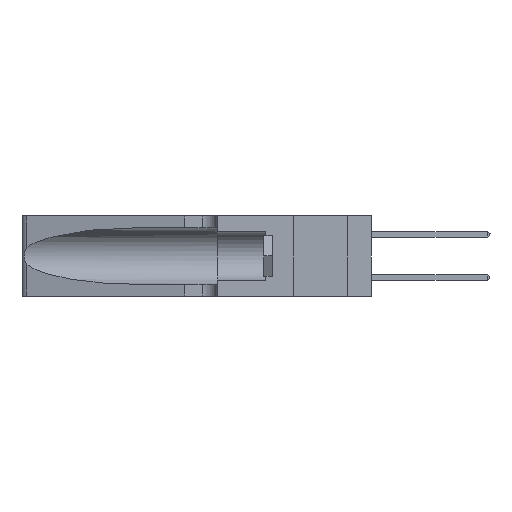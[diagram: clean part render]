
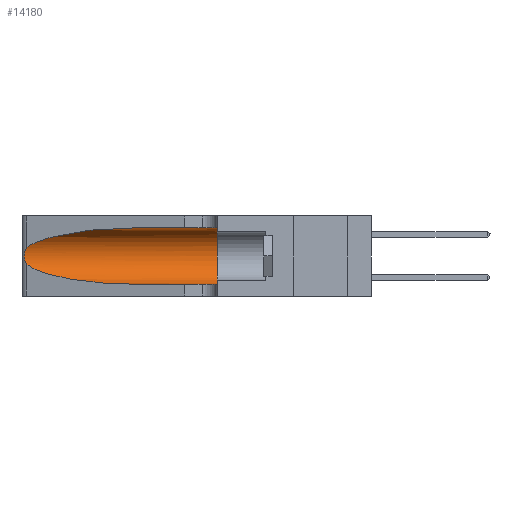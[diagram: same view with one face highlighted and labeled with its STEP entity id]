
A CAD part, left-side view. The second image highlights one B-rep face of the part: STEP entity #14180.
In plain terms, the highlighted cylindrical face has radius 3.308 mm (diameter 6.617 mm), a partial arc.
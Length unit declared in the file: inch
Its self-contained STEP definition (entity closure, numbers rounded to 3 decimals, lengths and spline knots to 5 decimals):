
#201 = CARTESIAN_POINT ( 'NONE',  ( 0.25487, 1.22718, 0.22369 ) ) ;
#343 = CARTESIAN_POINT ( 'NONE',  ( 0.25789, 1.23486, 0.15765 ) ) ;
#1265 = CARTESIAN_POINT ( 'NONE',  ( 0.18966, 0.96281, 0.31525 ) ) ;
#2607 = CARTESIAN_POINT ( 'NONE',  ( 0.1305, 0.72297, 0.05475 ) ) ;
#2677 = VERTEX_POINT ( 'NONE', #3471 ) ;
#3279 = VERTEX_POINT ( 'NONE', #37789 ) ;
#3471 = CARTESIAN_POINT ( 'NONE',  ( 0.25487, 1.22718, 0.14631 ) ) ;
#3675 = CARTESIAN_POINT ( 'NONE',  ( 0.25555, 1.22994, 0.2215 ) ) ;
#3824 = CARTESIAN_POINT ( 'NONE',  ( 0.25555, 1.22993, 0.14849 ) ) ;
#5487 = CARTESIAN_POINT ( 'NONE',  ( 0.1305, 0.72297, 0.05475 ) ) ;
#6386 = DIRECTION ( 'NONE',  ( 0., -1., 0. ) ) ;
#7537 =( BOUNDED_CURVE ( )  B_SPLINE_CURVE ( 3, ( #28730, #1265, #35580, #15104 ),
 .UNSPECIFIED., .F., .F. ) 
 B_SPLINE_CURVE_WITH_KNOTS ( ( 4, 4 ),
 ( 1.5708, 2.84003 ),
 .UNSPECIFIED. ) 
 CURVE ( )  GEOMETRIC_REPRESENTATION_ITEM ( )  RATIONAL_B_SPLINE_CURVE ( ( 1., 0.87, 0.87, 1. ) ) 
 REPRESENTATION_ITEM ( '' )  );
#7793 = VERTEX_POINT ( 'NONE', #5487 ) ;
#7988 = EDGE_CURVE ( 'NONE', #42000, #37596, #18874, .T. ) ;
#10595 = CARTESIAN_POINT ( 'NONE',  ( 0.25787, 1.23484, 0.2124 ) ) ;
#12994 = FACE_OUTER_BOUND ( 'NONE', #30036, .T. ) ;
#14050 = CARTESIAN_POINT ( 'NONE',  ( 0.26018, 1.23835, 0.19895 ) ) ;
#14180 = ADVANCED_FACE ( 'NONE', ( #12994 ), #29038, .F. ) ;
#15104 = CARTESIAN_POINT ( 'NONE',  ( 0.25487, 1.22718, 0.22369 ) ) ;
#16014 = ORIENTED_EDGE ( 'NONE', *, *, #7988, .F. ) ;
#16285 = CARTESIAN_POINT ( 'NONE',  ( 0.2373, 1.15595, 0.08982 ) ) ;
#16546 = DIRECTION ( 'NONE',  ( 0., 0., -1. ) ) ;
#17199 = CARTESIAN_POINT ( 'NONE',  ( 0.1305, 0.35, 0.185 ) ) ;
#17522 = CARTESIAN_POINT ( 'NONE',  ( 0.26075, 1.23896, 0.178 ) ) ;
#17794 = EDGE_CURVE ( 'NONE', #37596, #3279, #40691, .T. ) ;
#18858 = EDGE_CURVE ( 'NONE', #7793, #3279, #25089, .T. ) ;
#18874 = LINE ( 'NONE', #30385, #25849 ) ;
#19587 = ORIENTED_EDGE ( 'NONE', *, *, #18858, .T. ) ;
#20236 =( BOUNDED_CURVE ( )  B_SPLINE_CURVE ( 3, ( #40221, #16285, #23189, #2607 ),
 .UNSPECIFIED., .F., .F. ) 
 B_SPLINE_CURVE_WITH_KNOTS ( ( 4, 4 ),
 ( 3.44316, 4.71239 ),
 .UNSPECIFIED. ) 
 CURVE ( )  GEOMETRIC_REPRESENTATION_ITEM ( )  RATIONAL_B_SPLINE_CURVE ( ( 1., 0.87, 0.87, 1. ) ) 
 REPRESENTATION_ITEM ( '' )  );
#20478 = AXIS2_PLACEMENT_3D ( 'NONE', #17199, #41097, #20645 ) ;
#20645 = DIRECTION ( 'NONE',  ( 0., 0., 1. ) ) ;
#20982 = CARTESIAN_POINT ( 'NONE',  ( 0.25856, 1.23593, 0.16098 ) ) ;
#21178 = ORIENTED_EDGE ( 'NONE', *, *, #35497, .T. ) ;
#22624 = ORIENTED_EDGE ( 'NONE', *, *, #43214, .T. ) ;
#23189 = CARTESIAN_POINT ( 'NONE',  ( 0.18966, 0.96281, 0.05475 ) ) ;
#24013 = VECTOR ( 'NONE', #33083, 39.37008 ) ;
#24325 = VERTEX_POINT ( 'NONE', #35336 ) ;
#24407 = CARTESIAN_POINT ( 'NONE',  ( 0.25639, 1.23186, 0.15144 ) ) ;
#25089 = LINE ( 'NONE', #40000, #24013 ) ;
#25849 = VECTOR ( 'NONE', #6386, 39.37008 ) ;
#27438 = ORIENTED_EDGE ( 'NONE', *, *, #42780, .T. ) ;
#27531 = AXIS2_PLACEMENT_3D ( 'NONE', #40328, #36991, #16546 ) ;
#27833 = CARTESIAN_POINT ( 'NONE',  ( 0.25487, 1.22718, 0.14631 ) ) ;
#28152 = B_SPLINE_CURVE_WITH_KNOTS ( 'NONE', 3,
 ( #201, #3675, #31092, #10595, #34537, #14050, #37963, #17522, #41417, #20982, #343, #24407, #3824, #27833 ),
 .UNSPECIFIED., .F., .F.,
 ( 4, 2, 2, 2, 2, 2, 4 ),
 ( 0., 0.00027, 0.00053, 0.00107, 0.0016, 0.00187, 0.00214 ),
 .UNSPECIFIED. ) ;
#28730 = CARTESIAN_POINT ( 'NONE',  ( 0.1305, 0.72297, 0.31525 ) ) ;
#29038 = CYLINDRICAL_SURFACE ( 'NONE', #27531, 0.13025 ) ;
#30036 = EDGE_LOOP ( 'NONE', ( #21178, #27438, #22624, #19587, #35735, #16014 ) ) ;
#30385 = CARTESIAN_POINT ( 'NONE',  ( 0.1305, 1.61858, 0.31525 ) ) ;
#31092 = CARTESIAN_POINT ( 'NONE',  ( 0.25639, 1.23184, 0.21858 ) ) ;
#33083 = DIRECTION ( 'NONE',  ( 0., -1., 0. ) ) ;
#33242 = CARTESIAN_POINT ( 'NONE',  ( 0.1305, 0.72297, 0.31525 ) ) ;
#34537 = CARTESIAN_POINT ( 'NONE',  ( 0.25854, 1.2359, 0.20912 ) ) ;
#35336 = CARTESIAN_POINT ( 'NONE',  ( 0.25487, 1.22718, 0.22369 ) ) ;
#35497 = EDGE_CURVE ( 'NONE', #42000, #24325, #7537, .T. ) ;
#35580 = CARTESIAN_POINT ( 'NONE',  ( 0.2373, 1.15595, 0.28018 ) ) ;
#35735 = ORIENTED_EDGE ( 'NONE', *, *, #17794, .F. ) ;
#36991 = DIRECTION ( 'NONE',  ( 0., -1., 0. ) ) ;
#37596 = VERTEX_POINT ( 'NONE', #40446 ) ;
#37789 = CARTESIAN_POINT ( 'NONE',  ( 0.1305, 0.35, 0.05475 ) ) ;
#37963 = CARTESIAN_POINT ( 'NONE',  ( 0.26075, 1.23896, 0.19203 ) ) ;
#40000 = CARTESIAN_POINT ( 'NONE',  ( 0.1305, 1.61858, 0.05475 ) ) ;
#40221 = CARTESIAN_POINT ( 'NONE',  ( 0.25487, 1.22718, 0.14631 ) ) ;
#40328 = CARTESIAN_POINT ( 'NONE',  ( 0.1305, 1.61858, 0.185 ) ) ;
#40446 = CARTESIAN_POINT ( 'NONE',  ( 0.1305, 0.35, 0.31525 ) ) ;
#40691 = CIRCLE ( 'NONE', #20478, 0.13025 ) ;
#41097 = DIRECTION ( 'NONE',  ( 0., 1., 0. ) ) ;
#41417 = CARTESIAN_POINT ( 'NONE',  ( 0.26017, 1.23833, 0.17102 ) ) ;
#42000 = VERTEX_POINT ( 'NONE', #33242 ) ;
#42780 = EDGE_CURVE ( 'NONE', #24325, #2677, #28152, .T. ) ;
#43214 = EDGE_CURVE ( 'NONE', #2677, #7793, #20236, .T. ) ;
